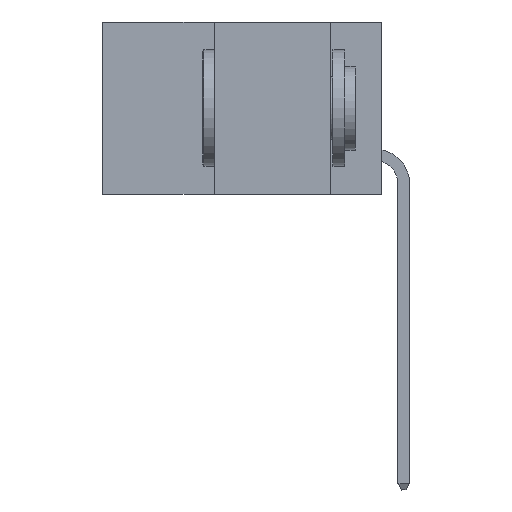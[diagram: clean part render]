
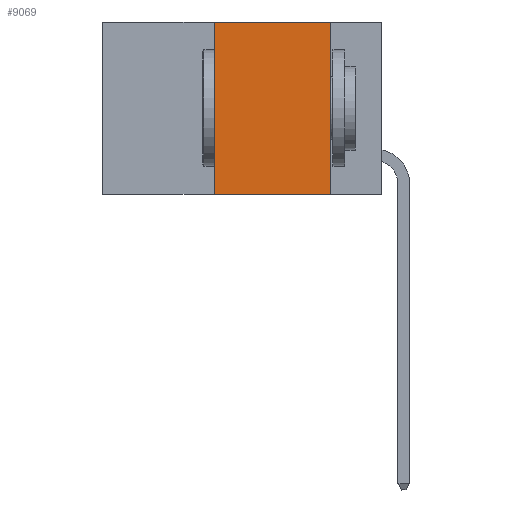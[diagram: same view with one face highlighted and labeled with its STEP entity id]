
A CAD part, left-side view. The second image highlights one B-rep face of the part: STEP entity #9069.
In plain terms, the highlighted planar face has unit normal (-1, 0, 0).
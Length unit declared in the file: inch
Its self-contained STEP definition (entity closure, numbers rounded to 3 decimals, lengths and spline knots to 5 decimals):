
#152 = LINE ( 'NONE', #223, #10784 ) ;
#223 = CARTESIAN_POINT ( 'NONE',  ( 0., 0.11, 0. ) ) ;
#401 = ORIENTED_EDGE ( 'NONE', *, *, #9448, .F. ) ;
#1508 = EDGE_CURVE ( 'NONE', #11939, #11446, #13021, .T. ) ;
#1518 = EDGE_LOOP ( 'NONE', ( #8387, #401, #2740, #13074 ) ) ;
#1787 = EDGE_CURVE ( 'NONE', #4917, #11446, #152, .T. ) ;
#2105 = CARTESIAN_POINT ( 'NONE',  ( 0., 0.11, 0. ) ) ;
#2158 = CARTESIAN_POINT ( 'NONE',  ( 0., 0.36, -0.37 ) ) ;
#2281 = VECTOR ( 'NONE', #9387, 39.37008 ) ;
#2740 = ORIENTED_EDGE ( 'NONE', *, *, #5404, .F. ) ;
#3127 = VECTOR ( 'NONE', #4040, 39.37008 ) ;
#4040 = DIRECTION ( 'NONE',  ( 0., 0., 1. ) ) ;
#4917 = VERTEX_POINT ( 'NONE', #2105 ) ;
#5150 = CARTESIAN_POINT ( 'NONE',  ( 0., 0.6, 0. ) ) ;
#5396 = PLANE ( 'NONE',  #11114 ) ;
#5404 = EDGE_CURVE ( 'NONE', #11939, #13115, #11328, .T. ) ;
#6275 = DIRECTION ( 'NONE',  ( 0., 0., -1. ) ) ;
#6370 = DIRECTION ( 'NONE',  ( 1., 0., 0. ) ) ;
#7486 = DIRECTION ( 'NONE',  ( 0., 0., -1. ) ) ;
#7767 = LINE ( 'NONE', #5150, #2281 ) ;
#8387 = ORIENTED_EDGE ( 'NONE', *, *, #1787, .F. ) ;
#8510 = VECTOR ( 'NONE', #12988, 39.37008 ) ;
#8565 = FACE_OUTER_BOUND ( 'NONE', #1518, .T. ) ;
#9069 = ADVANCED_FACE ( 'NONE', ( #8565 ), #5396, .F. ) ;
#9387 = DIRECTION ( 'NONE',  ( 0., -1., 0. ) ) ;
#9448 = EDGE_CURVE ( 'NONE', #13115, #4917, #7767, .T. ) ;
#9761 = CARTESIAN_POINT ( 'NONE',  ( 0., 0.11, -0.37 ) ) ;
#10403 = CARTESIAN_POINT ( 'NONE',  ( 0., 0.6, 0. ) ) ;
#10784 = VECTOR ( 'NONE', #6275, 39.37008 ) ;
#11114 = AXIS2_PLACEMENT_3D ( 'NONE', #10403, #6370, #7486 ) ;
#11328 = LINE ( 'NONE', #11738, #3127 ) ;
#11446 = VERTEX_POINT ( 'NONE', #9761 ) ;
#11738 = CARTESIAN_POINT ( 'NONE',  ( 0., 0.36, 0. ) ) ;
#11790 = CARTESIAN_POINT ( 'NONE',  ( 0., 0.36, 0. ) ) ;
#11841 = CARTESIAN_POINT ( 'NONE',  ( 0., 0.6, -0.37 ) ) ;
#11939 = VERTEX_POINT ( 'NONE', #2158 ) ;
#12988 = DIRECTION ( 'NONE',  ( 0., -1., 0. ) ) ;
#13021 = LINE ( 'NONE', #11841, #8510 ) ;
#13074 = ORIENTED_EDGE ( 'NONE', *, *, #1508, .T. ) ;
#13115 = VERTEX_POINT ( 'NONE', #11790 ) ;
